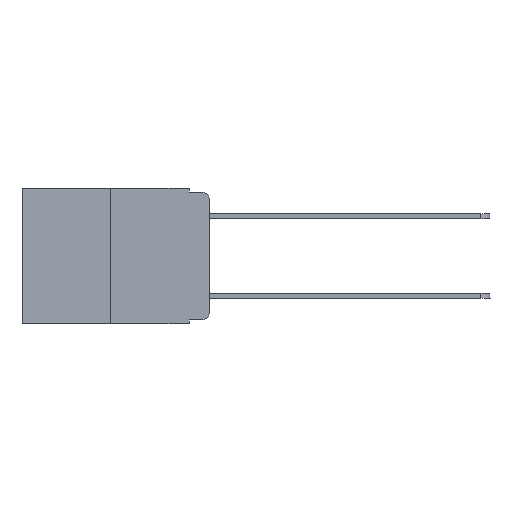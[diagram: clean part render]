
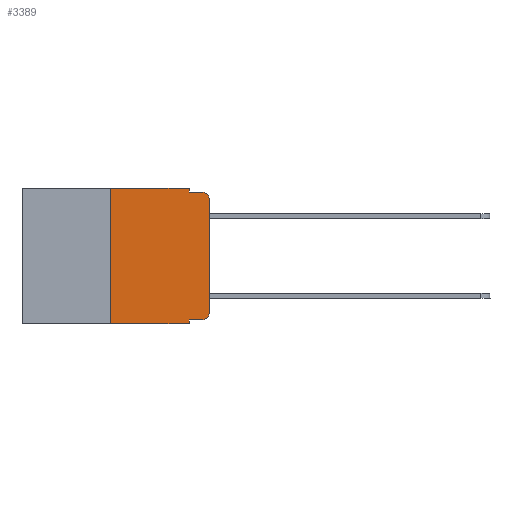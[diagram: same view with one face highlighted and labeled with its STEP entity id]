
A CAD part, left-side view. The second image highlights one B-rep face of the part: STEP entity #3389.
In plain terms, the highlighted planar face has unit normal (-1, 0, 0).
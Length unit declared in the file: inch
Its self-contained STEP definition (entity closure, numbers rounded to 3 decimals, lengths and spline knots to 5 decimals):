
#73 = ORIENTED_EDGE ( 'NONE', *, *, #8103, .F. ) ;
#259 = DIRECTION ( 'NONE',  ( -1., 0., 0. ) ) ;
#312 = EDGE_CURVE ( 'NONE', #10073, #2285, #488, .T. ) ;
#325 = CARTESIAN_POINT ( 'NONE',  ( 0., 0.25, 0. ) ) ;
#479 = DIRECTION ( 'NONE',  ( -1., 0., 0. ) ) ;
#488 = LINE ( 'NONE', #3075, #5935 ) ;
#540 = CARTESIAN_POINT ( 'NONE',  ( 0., 0.02, -0.333 ) ) ;
#1170 = VECTOR ( 'NONE', #7049, 39.37008 ) ;
#1349 = VERTEX_POINT ( 'NONE', #9182 ) ;
#1496 = EDGE_CURVE ( 'NONE', #1349, #6111, #5189, .T. ) ;
#1890 = ORIENTED_EDGE ( 'NONE', *, *, #5049, .T. ) ;
#1919 = DIRECTION ( 'NONE',  ( 0., 0., -1. ) ) ;
#2012 = VECTOR ( 'NONE', #2054, 39.37008 ) ;
#2054 = DIRECTION ( 'NONE',  ( 0., 0., -1. ) ) ;
#2077 = DIRECTION ( 'NONE',  ( 0., 0., -1. ) ) ;
#2107 = EDGE_CURVE ( 'NONE', #7929, #6166, #4512, .T. ) ;
#2285 = VERTEX_POINT ( 'NONE', #7972 ) ;
#2555 = LINE ( 'NONE', #3215, #8887 ) ;
#2625 = VERTEX_POINT ( 'NONE', #3212 ) ;
#2761 = CARTESIAN_POINT ( 'NONE',  ( 0., 0.02, -0.03 ) ) ;
#2834 = ORIENTED_EDGE ( 'NONE', *, *, #3337, .T. ) ;
#2857 = DIRECTION ( 'NONE',  ( 0., 0., 1. ) ) ;
#3075 = CARTESIAN_POINT ( 'NONE',  ( 0., 0., 0. ) ) ;
#3212 = CARTESIAN_POINT ( 'NONE',  ( 0., 0.051, 0. ) ) ;
#3215 = CARTESIAN_POINT ( 'NONE',  ( 0., 0.051, -0.333 ) ) ;
#3229 = CARTESIAN_POINT ( 'NONE',  ( 0., 0.473, 0. ) ) ;
#3274 = ORIENTED_EDGE ( 'NONE', *, *, #5694, .F. ) ;
#3337 = EDGE_CURVE ( 'NONE', #6002, #10073, #9796, .T. ) ;
#3389 = ADVANCED_FACE ( 'NONE', ( #4726 ), #9831, .F. ) ;
#3661 = VERTEX_POINT ( 'NONE', #5390 ) ;
#3664 = CARTESIAN_POINT ( 'NONE',  ( 0., 0.051, 0. ) ) ;
#3686 = CARTESIAN_POINT ( 'NONE',  ( 0., 0.051, -0.01 ) ) ;
#3930 = VECTOR ( 'NONE', #4208, 39.37008 ) ;
#3950 = DIRECTION ( 'NONE',  ( 0., 0., -1. ) ) ;
#4208 = DIRECTION ( 'NONE',  ( 0., 0., -1. ) ) ;
#4249 = CARTESIAN_POINT ( 'NONE',  ( 0., 0.051, -0.343 ) ) ;
#4512 = LINE ( 'NONE', #3686, #1170 ) ;
#4671 = AXIS2_PLACEMENT_3D ( 'NONE', #8059, #479, #3950 ) ;
#4726 = FACE_OUTER_BOUND ( 'NONE', #9759, .T. ) ;
#5049 = EDGE_CURVE ( 'NONE', #1349, #7259, #10427, .T. ) ;
#5189 = LINE ( 'NONE', #325, #6623 ) ;
#5390 = CARTESIAN_POINT ( 'NONE',  ( 0., 0.051, -0.333 ) ) ;
#5694 = EDGE_CURVE ( 'NONE', #2625, #7929, #8186, .T. ) ;
#5935 = VECTOR ( 'NONE', #2857, 39.37008 ) ;
#6002 = VERTEX_POINT ( 'NONE', #540 ) ;
#6111 = VERTEX_POINT ( 'NONE', #10012 ) ;
#6166 = VERTEX_POINT ( 'NONE', #7449 ) ;
#6252 = LINE ( 'NONE', #3664, #2012 ) ;
#6285 = CARTESIAN_POINT ( 'NONE',  ( 0., 0.473, 0. ) ) ;
#6519 = ORIENTED_EDGE ( 'NONE', *, *, #8529, .T. ) ;
#6602 = DIRECTION ( 'NONE',  ( 0., -1., 0. ) ) ;
#6604 = ORIENTED_EDGE ( 'NONE', *, *, #312, .T. ) ;
#6623 = VECTOR ( 'NONE', #7792, 39.37008 ) ;
#6773 = CIRCLE ( 'NONE', #7489, 0.02 ) ;
#7039 = EDGE_CURVE ( 'NONE', #3661, #7259, #6252, .T. ) ;
#7049 = DIRECTION ( 'NONE',  ( 0., -1., 0. ) ) ;
#7178 = ORIENTED_EDGE ( 'NONE', *, *, #2107, .F. ) ;
#7259 = VERTEX_POINT ( 'NONE', #4249 ) ;
#7311 = AXIS2_PLACEMENT_3D ( 'NONE', #6285, #7994, #2077 ) ;
#7449 = CARTESIAN_POINT ( 'NONE',  ( 0., 0.02, -0.01 ) ) ;
#7489 = AXIS2_PLACEMENT_3D ( 'NONE', #2761, #259, #1919 ) ;
#7792 = DIRECTION ( 'NONE',  ( 0., 0., 1. ) ) ;
#7929 = VERTEX_POINT ( 'NONE', #10336 ) ;
#7955 = ORIENTED_EDGE ( 'NONE', *, *, #7039, .F. ) ;
#7972 = CARTESIAN_POINT ( 'NONE',  ( 0., 0., -0.03 ) ) ;
#7994 = DIRECTION ( 'NONE',  ( 1., 0., 0. ) ) ;
#8059 = CARTESIAN_POINT ( 'NONE',  ( 0., 0.02, -0.313 ) ) ;
#8103 = EDGE_CURVE ( 'NONE', #6111, #2625, #8278, .T. ) ;
#8182 = VECTOR ( 'NONE', #8703, 39.37008 ) ;
#8186 = LINE ( 'NONE', #8255, #3930 ) ;
#8255 = CARTESIAN_POINT ( 'NONE',  ( 0., 0.051, 0. ) ) ;
#8278 = LINE ( 'NONE', #3229, #8399 ) ;
#8399 = VECTOR ( 'NONE', #6602, 39.37008 ) ;
#8529 = EDGE_CURVE ( 'NONE', #3661, #6002, #2555, .T. ) ;
#8597 = CARTESIAN_POINT ( 'NONE',  ( 0., 0., -0.313 ) ) ;
#8608 = CARTESIAN_POINT ( 'NONE',  ( 0., 0.473, -0.343 ) ) ;
#8703 = DIRECTION ( 'NONE',  ( 0., -1., 0. ) ) ;
#8887 = VECTOR ( 'NONE', #9978, 39.37008 ) ;
#9126 = ORIENTED_EDGE ( 'NONE', *, *, #1496, .F. ) ;
#9182 = CARTESIAN_POINT ( 'NONE',  ( 0., 0.25, -0.343 ) ) ;
#9206 = EDGE_CURVE ( 'NONE', #2285, #6166, #6773, .T. ) ;
#9759 = EDGE_LOOP ( 'NONE', ( #6604, #10932, #7178, #3274, #73, #9126, #1890, #7955, #6519, #2834 ) ) ;
#9796 = CIRCLE ( 'NONE', #4671, 0.02 ) ;
#9831 = PLANE ( 'NONE',  #7311 ) ;
#9978 = DIRECTION ( 'NONE',  ( 0., -1., 0. ) ) ;
#10012 = CARTESIAN_POINT ( 'NONE',  ( 0., 0.25, 0. ) ) ;
#10073 = VERTEX_POINT ( 'NONE', #8597 ) ;
#10336 = CARTESIAN_POINT ( 'NONE',  ( 0., 0.051, -0.01 ) ) ;
#10427 = LINE ( 'NONE', #8608, #8182 ) ;
#10932 = ORIENTED_EDGE ( 'NONE', *, *, #9206, .T. ) ;
